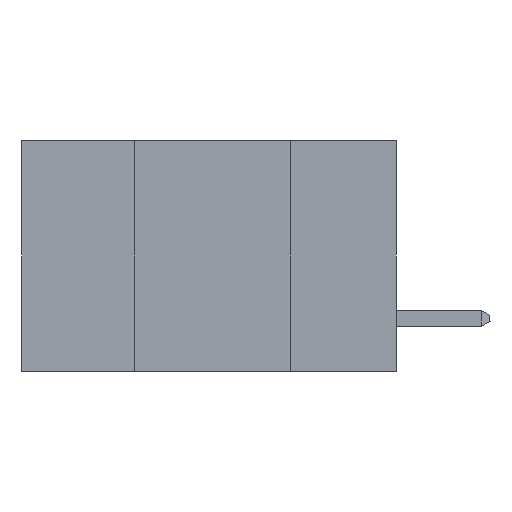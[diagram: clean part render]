
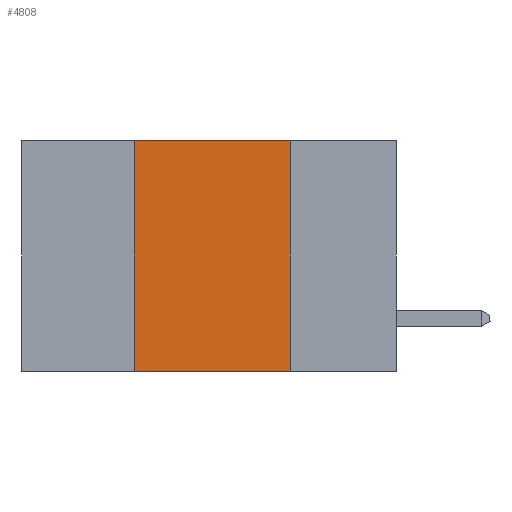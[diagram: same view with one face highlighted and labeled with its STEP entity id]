
A CAD part, left-side view. The second image highlights one B-rep face of the part: STEP entity #4808.
In plain terms, the highlighted planar face has unit normal (-1, 0, 0).
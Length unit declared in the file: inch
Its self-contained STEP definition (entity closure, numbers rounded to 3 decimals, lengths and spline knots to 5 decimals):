
#762 = DIRECTION ( 'NONE',  ( 0., -1., 0. ) ) ;
#1194 = DIRECTION ( 'NONE',  ( 0., 0., 1. ) ) ;
#1650 = EDGE_CURVE ( 'NONE', #12255, #15599, #6203, .T. ) ;
#1682 = EDGE_LOOP ( 'NONE', ( #16053, #7578, #4375, #1995 ) ) ;
#1995 = ORIENTED_EDGE ( 'NONE', *, *, #11977, .T. ) ;
#2443 = CARTESIAN_POINT ( 'NONE',  ( 0., 0.6, -0.37 ) ) ;
#3609 = DIRECTION ( 'NONE',  ( 0., 0., -1. ) ) ;
#3652 = EDGE_CURVE ( 'NONE', #11597, #13473, #5063, .T. ) ;
#3709 = FACE_OUTER_BOUND ( 'NONE', #1682, .T. ) ;
#4375 = ORIENTED_EDGE ( 'NONE', *, *, #1650, .F. ) ;
#4423 = VECTOR ( 'NONE', #10267, 39.37008 ) ;
#4808 = ADVANCED_FACE ( 'NONE', ( #3709 ), #8627, .F. ) ;
#4909 = CARTESIAN_POINT ( 'NONE',  ( 0., 0.17, 0. ) ) ;
#4969 = DIRECTION ( 'NONE',  ( 0., 0., -1. ) ) ;
#5063 = LINE ( 'NONE', #4909, #5492 ) ;
#5446 = EDGE_CURVE ( 'NONE', #15599, #11597, #9092, .T. ) ;
#5492 = VECTOR ( 'NONE', #4969, 39.37008 ) ;
#6103 = CARTESIAN_POINT ( 'NONE',  ( 0., 0.6, 0. ) ) ;
#6203 = LINE ( 'NONE', #11746, #16422 ) ;
#6618 = VECTOR ( 'NONE', #762, 39.37008 ) ;
#7420 = CARTESIAN_POINT ( 'NONE',  ( 0., 0.6, 0. ) ) ;
#7475 = DIRECTION ( 'NONE',  ( 1., 0., 0. ) ) ;
#7578 = ORIENTED_EDGE ( 'NONE', *, *, #5446, .F. ) ;
#8004 = CARTESIAN_POINT ( 'NONE',  ( 0., 0.17, 0. ) ) ;
#8378 = LINE ( 'NONE', #2443, #4423 ) ;
#8627 = PLANE ( 'NONE',  #16375 ) ;
#9092 = LINE ( 'NONE', #6103, #6618 ) ;
#9577 = CARTESIAN_POINT ( 'NONE',  ( 0., 0.42, -0.37 ) ) ;
#10267 = DIRECTION ( 'NONE',  ( 0., -1., 0. ) ) ;
#11597 = VERTEX_POINT ( 'NONE', #8004 ) ;
#11746 = CARTESIAN_POINT ( 'NONE',  ( 0., 0.42, 0. ) ) ;
#11827 = CARTESIAN_POINT ( 'NONE',  ( 0., 0.42, 0. ) ) ;
#11977 = EDGE_CURVE ( 'NONE', #12255, #13473, #8378, .T. ) ;
#12229 = CARTESIAN_POINT ( 'NONE',  ( 0., 0.17, -0.37 ) ) ;
#12255 = VERTEX_POINT ( 'NONE', #9577 ) ;
#13473 = VERTEX_POINT ( 'NONE', #12229 ) ;
#15599 = VERTEX_POINT ( 'NONE', #11827 ) ;
#16053 = ORIENTED_EDGE ( 'NONE', *, *, #3652, .F. ) ;
#16375 = AXIS2_PLACEMENT_3D ( 'NONE', #7420, #7475, #3609 ) ;
#16422 = VECTOR ( 'NONE', #1194, 39.37008 ) ;
